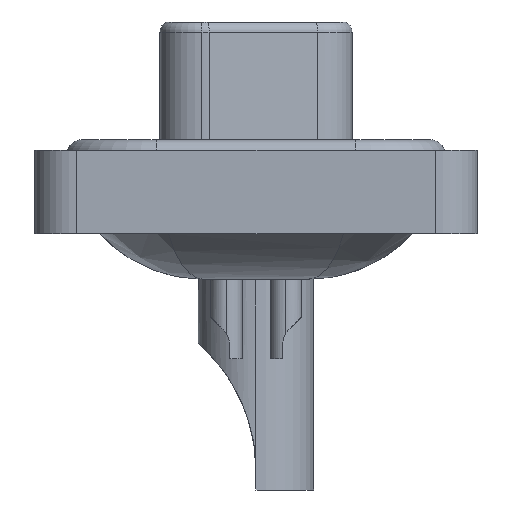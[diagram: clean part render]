
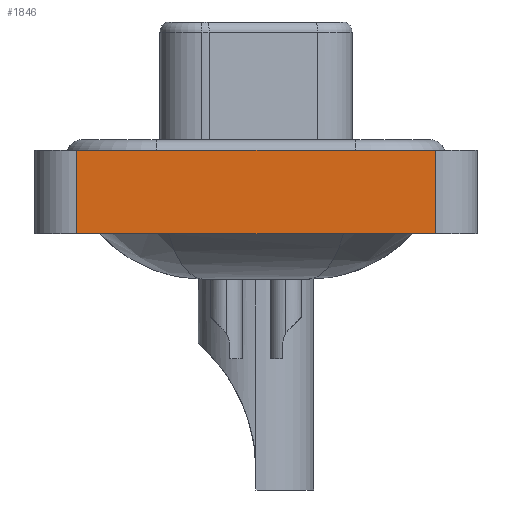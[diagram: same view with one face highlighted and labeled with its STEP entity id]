
A CAD part, left-side view. The second image highlights one B-rep face of the part: STEP entity #1846.
In plain terms, the highlighted planar face has unit normal (-1, 0, 0).
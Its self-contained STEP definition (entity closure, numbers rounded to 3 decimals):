
#3 = EDGE_CURVE ( 'NONE', #11751, #3467, #15433, .T. ) ;
#194 = DIRECTION ( 'NONE',  ( 0., -1., 0. ) ) ;
#537 = DIRECTION ( 'NONE',  ( -1., 0., 0. ) ) ;
#1846 = ADVANCED_FACE ( 'NONE', ( #3320 ), #16863, .T. ) ;
#2005 = CARTESIAN_POINT ( 'NONE',  ( -7.25, 8.55, -3.6 ) ) ;
#2532 = EDGE_LOOP ( 'NONE', ( #17343, #5811, #2752, #7699 ) ) ;
#2752 = ORIENTED_EDGE ( 'NONE', *, *, #3, .F. ) ;
#2990 = CARTESIAN_POINT ( 'NONE',  ( -7.25, -8.55, 0.4 ) ) ;
#3165 = VERTEX_POINT ( 'NONE', #14998 ) ;
#3320 = FACE_OUTER_BOUND ( 'NONE', #2532, .T. ) ;
#3467 = VERTEX_POINT ( 'NONE', #13238 ) ;
#3512 = CARTESIAN_POINT ( 'NONE',  ( -7.25, -8.55, -3.6 ) ) ;
#4779 = CARTESIAN_POINT ( 'NONE',  ( -7.25, 8.55, -3.6 ) ) ;
#5811 = ORIENTED_EDGE ( 'NONE', *, *, #6174, .F. ) ;
#6174 = EDGE_CURVE ( 'NONE', #3467, #7435, #16251, .T. ) ;
#6203 = DIRECTION ( 'NONE',  ( 0., 0., 1. ) ) ;
#6832 = VECTOR ( 'NONE', #194, 1000. ) ;
#7435 = VERTEX_POINT ( 'NONE', #2990 ) ;
#7471 = DIRECTION ( 'NONE',  ( 0., 0., 1. ) ) ;
#7699 = ORIENTED_EDGE ( 'NONE', *, *, #9845, .T. ) ;
#8575 = LINE ( 'NONE', #13995, #6832 ) ;
#9845 = EDGE_CURVE ( 'NONE', #11751, #3165, #8575, .T. ) ;
#10213 = VECTOR ( 'NONE', #15540, 1000. ) ;
#11751 = VERTEX_POINT ( 'NONE', #2005 ) ;
#12052 = VECTOR ( 'NONE', #6203, 1000. ) ;
#12718 = CARTESIAN_POINT ( 'NONE',  ( -7.25, -8.55, -3.6 ) ) ;
#13001 = LINE ( 'NONE', #3512, #12052 ) ;
#13238 = CARTESIAN_POINT ( 'NONE',  ( -7.25, 8.55, 0.4 ) ) ;
#13995 = CARTESIAN_POINT ( 'NONE',  ( -7.25, -8.55, -3.6 ) ) ;
#14282 = VECTOR ( 'NONE', #15270, 1000. ) ;
#14995 = CARTESIAN_POINT ( 'NONE',  ( -7.25, -8.55, 0.4 ) ) ;
#14998 = CARTESIAN_POINT ( 'NONE',  ( -7.25, -8.55, -3.6 ) ) ;
#15270 = DIRECTION ( 'NONE',  ( 0., -1., 0. ) ) ;
#15433 = LINE ( 'NONE', #4779, #10213 ) ;
#15540 = DIRECTION ( 'NONE',  ( 0., 0., 1. ) ) ;
#15757 = AXIS2_PLACEMENT_3D ( 'NONE', #12718, #537, #7471 ) ;
#16251 = LINE ( 'NONE', #14995, #14282 ) ;
#16863 = PLANE ( 'NONE',  #15757 ) ;
#17343 = ORIENTED_EDGE ( 'NONE', *, *, #17351, .T. ) ;
#17351 = EDGE_CURVE ( 'NONE', #3165, #7435, #13001, .T. ) ;
